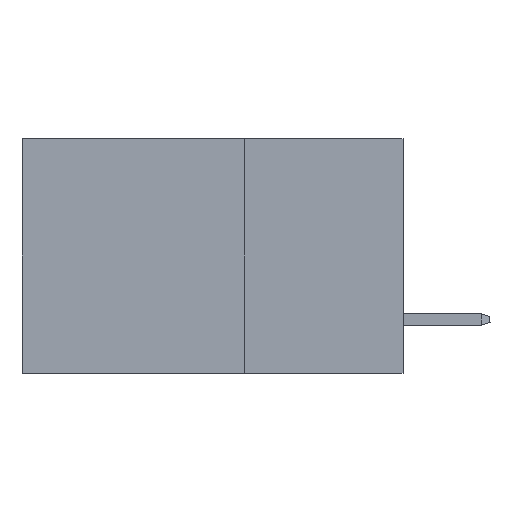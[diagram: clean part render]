
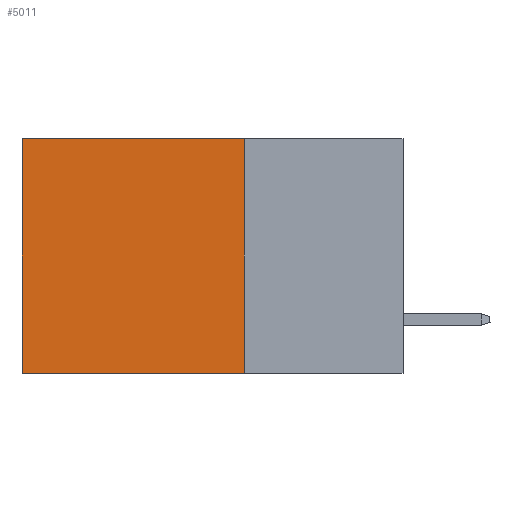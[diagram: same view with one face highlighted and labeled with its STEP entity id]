
A CAD part, left-side view. The second image highlights one B-rep face of the part: STEP entity #5011.
In plain terms, the highlighted planar face has unit normal (-1, 0, 0).
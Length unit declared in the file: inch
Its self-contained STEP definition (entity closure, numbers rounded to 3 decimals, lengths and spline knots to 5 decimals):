
#473 = EDGE_CURVE ( 'NONE', #17274, #3558, #14965, .T. ) ;
#857 = EDGE_LOOP ( 'NONE', ( #2200, #10053, #11535, #18201 ) ) ;
#865 = VECTOR ( 'NONE', #4649, 39.37008 ) ;
#1403 = FACE_OUTER_BOUND ( 'NONE', #857, .T. ) ;
#2200 = ORIENTED_EDGE ( 'NONE', *, *, #473, .T. ) ;
#2704 = CARTESIAN_POINT ( 'NONE',  ( 0.2875, 0.25, 0. ) ) ;
#3558 = VERTEX_POINT ( 'NONE', #18221 ) ;
#4628 = AXIS2_PLACEMENT_3D ( 'NONE', #17593, #8622, #8424 ) ;
#4649 = DIRECTION ( 'NONE',  ( 0., 0., -1. ) ) ;
#5011 = ADVANCED_FACE ( 'NONE', ( #1403 ), #7176, .F. ) ;
#5096 = LINE ( 'NONE', #5277, #14692 ) ;
#5277 = CARTESIAN_POINT ( 'NONE',  ( 0.2875, 0.25, 0. ) ) ;
#7176 = PLANE ( 'NONE',  #4628 ) ;
#7359 = EDGE_CURVE ( 'NONE', #17632, #17274, #5096, .T. ) ;
#7667 = VECTOR ( 'NONE', #14510, 39.37008 ) ;
#8424 = DIRECTION ( 'NONE',  ( 0., 0., -1. ) ) ;
#8622 = DIRECTION ( 'NONE',  ( 1., 0., 0. ) ) ;
#8648 = LINE ( 'NONE', #2704, #8757 ) ;
#8757 = VECTOR ( 'NONE', #14592, 39.37008 ) ;
#10053 = ORIENTED_EDGE ( 'NONE', *, *, #10281, .F. ) ;
#10118 = CARTESIAN_POINT ( 'NONE',  ( 0.2875, 0.25, -0.37 ) ) ;
#10281 = EDGE_CURVE ( 'NONE', #12420, #3558, #12861, .T. ) ;
#10951 = CARTESIAN_POINT ( 'NONE',  ( 0.2875, 0.6, 0. ) ) ;
#11535 = ORIENTED_EDGE ( 'NONE', *, *, #17792, .F. ) ;
#12420 = VERTEX_POINT ( 'NONE', #18554 ) ;
#12861 = LINE ( 'NONE', #10118, #7667 ) ;
#14510 = DIRECTION ( 'NONE',  ( 0., 1., 0. ) ) ;
#14592 = DIRECTION ( 'NONE',  ( 0., 0., -1. ) ) ;
#14692 = VECTOR ( 'NONE', #17265, 39.37008 ) ;
#14965 = LINE ( 'NONE', #16455, #865 ) ;
#15281 = CARTESIAN_POINT ( 'NONE',  ( 0.2875, 0.25, 0. ) ) ;
#16455 = CARTESIAN_POINT ( 'NONE',  ( 0.2875, 0.6, 0. ) ) ;
#17265 = DIRECTION ( 'NONE',  ( 0., 1., 0. ) ) ;
#17274 = VERTEX_POINT ( 'NONE', #10951 ) ;
#17593 = CARTESIAN_POINT ( 'NONE',  ( 0.2875, 0.25, 0. ) ) ;
#17632 = VERTEX_POINT ( 'NONE', #15281 ) ;
#17792 = EDGE_CURVE ( 'NONE', #17632, #12420, #8648, .T. ) ;
#18201 = ORIENTED_EDGE ( 'NONE', *, *, #7359, .T. ) ;
#18221 = CARTESIAN_POINT ( 'NONE',  ( 0.2875, 0.6, -0.37 ) ) ;
#18554 = CARTESIAN_POINT ( 'NONE',  ( 0.2875, 0.25, -0.37 ) ) ;
